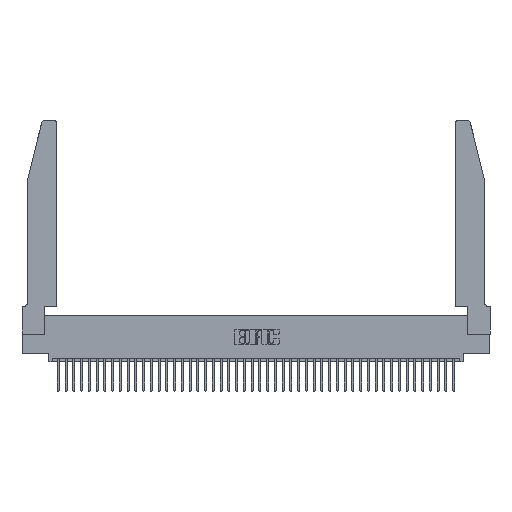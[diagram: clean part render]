
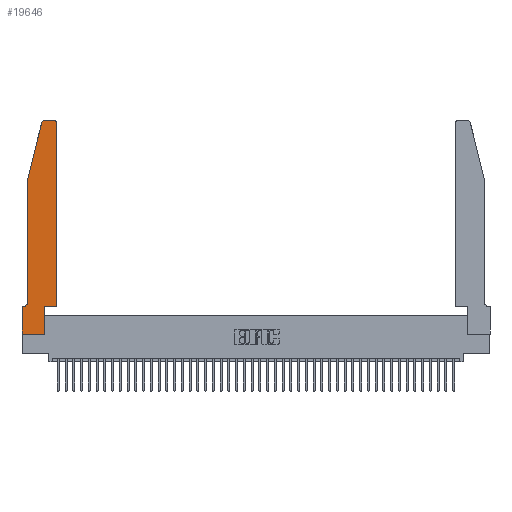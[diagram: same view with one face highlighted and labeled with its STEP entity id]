
A CAD part, top view. The second image highlights one B-rep face of the part: STEP entity #19646.
In plain terms, the highlighted planar face has unit normal (0, 0, 1).
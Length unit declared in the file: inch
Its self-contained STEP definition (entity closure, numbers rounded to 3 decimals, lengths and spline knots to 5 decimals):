
#25 = VERTEX_POINT ( 'NONE', #11263 ) ;
#620 = ORIENTED_EDGE ( 'NONE', *, *, #6630, .T. ) ;
#1118 = ORIENTED_EDGE ( 'NONE', *, *, #4806, .T. ) ;
#1131 = CARTESIAN_POINT ( 'NONE',  ( 0.284, 2.72, 0.37 ) ) ;
#1142 = VERTEX_POINT ( 'NONE', #27318 ) ;
#1952 = EDGE_CURVE ( 'NONE', #25, #10375, #27367, .T. ) ;
#2378 = CARTESIAN_POINT ( 'NONE',  ( 0.0055, 0.42, 0.37 ) ) ;
#2493 = DIRECTION ( 'NONE',  ( 0., 1., 0. ) ) ;
#3737 = CARTESIAN_POINT ( 'NONE',  ( 0.4505, 0.35, 0.37 ) ) ;
#4185 = LINE ( 'NONE', #23233, #31671 ) ;
#4429 = ORIENTED_EDGE ( 'NONE', *, *, #43973, .T. ) ;
#4659 = DIRECTION ( 'NONE',  ( 1., 0., 0. ) ) ;
#4806 = EDGE_CURVE ( 'NONE', #40997, #22156, #20809, .T. ) ;
#5314 = CARTESIAN_POINT ( 'NONE',  ( 0.0755, 0.42, 0.37 ) ) ;
#5592 = DIRECTION ( 'NONE',  ( 0., 0., 1. ) ) ;
#5885 = DIRECTION ( 'NONE',  ( -1., 0., 0. ) ) ;
#6110 = CARTESIAN_POINT ( 'NONE',  ( 0.4205, 2.75, 0.37 ) ) ;
#6630 = EDGE_CURVE ( 'NONE', #27160, #27197, #37423, .T. ) ;
#6637 = ORIENTED_EDGE ( 'NONE', *, *, #15648, .T. ) ;
#7489 = VECTOR ( 'NONE', #26339, 39.37008 ) ;
#8265 = VERTEX_POINT ( 'NONE', #15039 ) ;
#9916 = CARTESIAN_POINT ( 'NONE',  ( 0.4205, 2.72, 0.37 ) ) ;
#10375 = VERTEX_POINT ( 'NONE', #38596 ) ;
#10509 = CARTESIAN_POINT ( 'NONE',  ( 0.0055, 0.35, 0.37 ) ) ;
#11263 = CARTESIAN_POINT ( 'NONE',  ( 0.2865, 0.35, 0.37 ) ) ;
#11801 = AXIS2_PLACEMENT_3D ( 'NONE', #1131, #25325, #4659 ) ;
#12326 = CARTESIAN_POINT ( 'NONE',  ( 0.0755, 2., 0.37 ) ) ;
#12572 = ORIENTED_EDGE ( 'NONE', *, *, #19692, .T. ) ;
#12915 = CIRCLE ( 'NONE', #11801, 0.03 ) ;
#12938 = CIRCLE ( 'NONE', #37453, 0.07 ) ;
#13391 = DIRECTION ( 'NONE',  ( 1., 0., 0. ) ) ;
#13903 = VECTOR ( 'NONE', #43719, 39.37008 ) ;
#14495 = VECTOR ( 'NONE', #18804, 39.37008 ) ;
#14579 = VERTEX_POINT ( 'NONE', #31140 ) ;
#15039 = CARTESIAN_POINT ( 'NONE',  ( 0., 0., 0.37 ) ) ;
#15296 = CARTESIAN_POINT ( 'NONE',  ( 0., 0., 0.37 ) ) ;
#15579 = LINE ( 'NONE', #15296, #14495 ) ;
#15648 = EDGE_CURVE ( 'NONE', #1142, #25, #4185, .T. ) ;
#16338 = ORIENTED_EDGE ( 'NONE', *, *, #34377, .T. ) ;
#17294 = EDGE_CURVE ( 'NONE', #10375, #27160, #30537, .T. ) ;
#17990 = ORIENTED_EDGE ( 'NONE', *, *, #1952, .T. ) ;
#18002 = EDGE_LOOP ( 'NONE', ( #16338, #34565, #18514, #1118, #12572, #30870, #4429, #41938, #6637, #17990, #36149, #620 ) ) ;
#18247 = VECTOR ( 'NONE', #28002, 39.37008 ) ;
#18514 = ORIENTED_EDGE ( 'NONE', *, *, #37399, .T. ) ;
#18804 = DIRECTION ( 'NONE',  ( 1., 0., 0. ) ) ;
#19646 = ADVANCED_FACE ( 'NONE', ( #33335 ), #43134, .T. ) ;
#19670 = DIRECTION ( 'NONE',  ( 0., -1., 0. ) ) ;
#19692 = EDGE_CURVE ( 'NONE', #22156, #42935, #12938, .T. ) ;
#19751 = CARTESIAN_POINT ( 'NONE',  ( 0.4505, 2.72, 0.37 ) ) ;
#19980 = CARTESIAN_POINT ( 'NONE',  ( 0.0755, 0.35, 0.37 ) ) ;
#20809 = LINE ( 'NONE', #40023, #37840 ) ;
#22001 = LINE ( 'NONE', #19980, #13903 ) ;
#22156 = VERTEX_POINT ( 'NONE', #5314 ) ;
#22925 = CARTESIAN_POINT ( 'NONE',  ( 0., 0., 0.37 ) ) ;
#23233 = CARTESIAN_POINT ( 'NONE',  ( 0.2865, 0.35, 0.37 ) ) ;
#24454 = DIRECTION ( 'NONE',  ( 0., 1., 0. ) ) ;
#24850 = EDGE_CURVE ( 'NONE', #8265, #1142, #15579, .T. ) ;
#25325 = DIRECTION ( 'NONE',  ( 0., 0., 1. ) ) ;
#25566 = EDGE_CURVE ( 'NONE', #42935, #42576, #22001, .T. ) ;
#26339 = DIRECTION ( 'NONE',  ( 0., -1., 0. ) ) ;
#26532 = DIRECTION ( 'NONE',  ( 0., 0., -1. ) ) ;
#26885 = VECTOR ( 'NONE', #34096, 39.37008 ) ;
#26910 = AXIS2_PLACEMENT_3D ( 'NONE', #9916, #33935, #13391 ) ;
#27160 = VERTEX_POINT ( 'NONE', #19751 ) ;
#27197 = VERTEX_POINT ( 'NONE', #6110 ) ;
#27231 = CARTESIAN_POINT ( 'NONE',  ( 0.2605, 2.75, 0.37 ) ) ;
#27318 = CARTESIAN_POINT ( 'NONE',  ( 0.2865, 0., 0.37 ) ) ;
#27367 = LINE ( 'NONE', #34718, #18247 ) ;
#28002 = DIRECTION ( 'NONE',  ( 1., 0., 0. ) ) ;
#29442 = VECTOR ( 'NONE', #24454, 39.37008 ) ;
#29683 = DIRECTION ( 'NONE',  ( 1., 0., 0. ) ) ;
#30537 = LINE ( 'NONE', #3737, #29442 ) ;
#30870 = ORIENTED_EDGE ( 'NONE', *, *, #25566, .T. ) ;
#31140 = CARTESIAN_POINT ( 'NONE',  ( 0.25487, 2.72718, 0.37 ) ) ;
#31671 = VECTOR ( 'NONE', #2493, 39.37008 ) ;
#32813 = CARTESIAN_POINT ( 'NONE',  ( 0., 0.35, 0.37 ) ) ;
#33335 = FACE_OUTER_BOUND ( 'NONE', #18002, .T. ) ;
#33935 = DIRECTION ( 'NONE',  ( 0., 0., 1. ) ) ;
#34096 = DIRECTION ( 'NONE',  ( -1., 0., 0. ) ) ;
#34377 = EDGE_CURVE ( 'NONE', #27197, #35786, #35925, .T. ) ;
#34565 = ORIENTED_EDGE ( 'NONE', *, *, #38525, .T. ) ;
#34718 = CARTESIAN_POINT ( 'NONE',  ( 0.4505, 0.35, 0.37 ) ) ;
#35138 = VECTOR ( 'NONE', #39671, 39.37008 ) ;
#35167 = AXIS2_PLACEMENT_3D ( 'NONE', #32813, #5592, #29683 ) ;
#35786 = VERTEX_POINT ( 'NONE', #38335 ) ;
#35925 = LINE ( 'NONE', #27231, #26885 ) ;
#35932 = LINE ( 'NONE', #22925, #7489 ) ;
#36149 = ORIENTED_EDGE ( 'NONE', *, *, #17294, .T. ) ;
#36193 = LINE ( 'NONE', #12326, #35138 ) ;
#36475 = CARTESIAN_POINT ( 'NONE',  ( 0.0755, 2., 0.37 ) ) ;
#37399 = EDGE_CURVE ( 'NONE', #14579, #40997, #36193, .T. ) ;
#37423 = CIRCLE ( 'NONE', #26910, 0.03 ) ;
#37453 = AXIS2_PLACEMENT_3D ( 'NONE', #2378, #26532, #5885 ) ;
#37840 = VECTOR ( 'NONE', #19670, 39.37008 ) ;
#38335 = CARTESIAN_POINT ( 'NONE',  ( 0.284, 2.75, 0.37 ) ) ;
#38525 = EDGE_CURVE ( 'NONE', #35786, #14579, #12915, .T. ) ;
#38596 = CARTESIAN_POINT ( 'NONE',  ( 0.4505, 0.35, 0.37 ) ) ;
#39671 = DIRECTION ( 'NONE',  ( -0.239, -0.971, 0. ) ) ;
#40023 = CARTESIAN_POINT ( 'NONE',  ( 0.0755, 2., 0.37 ) ) ;
#40997 = VERTEX_POINT ( 'NONE', #36475 ) ;
#41938 = ORIENTED_EDGE ( 'NONE', *, *, #24850, .T. ) ;
#42576 = VERTEX_POINT ( 'NONE', #42902 ) ;
#42902 = CARTESIAN_POINT ( 'NONE',  ( 0., 0.35, 0.37 ) ) ;
#42935 = VERTEX_POINT ( 'NONE', #10509 ) ;
#43134 = PLANE ( 'NONE',  #35167 ) ;
#43719 = DIRECTION ( 'NONE',  ( -1., 0., 0. ) ) ;
#43973 = EDGE_CURVE ( 'NONE', #42576, #8265, #35932, .T. ) ;
